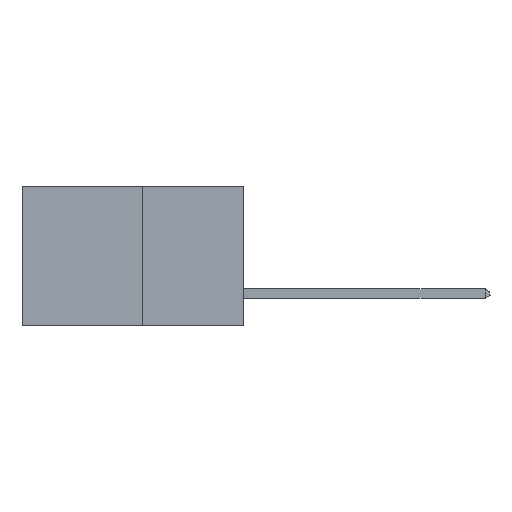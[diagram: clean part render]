
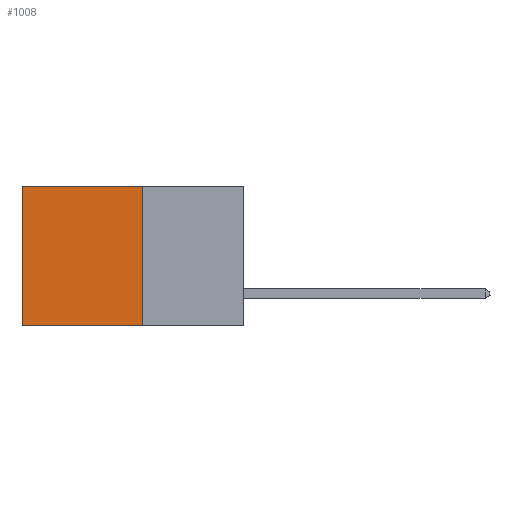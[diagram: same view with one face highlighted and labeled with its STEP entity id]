
A CAD part, left-side view. The second image highlights one B-rep face of the part: STEP entity #1008.
In plain terms, the highlighted planar face has unit normal (-1, 0, 0).
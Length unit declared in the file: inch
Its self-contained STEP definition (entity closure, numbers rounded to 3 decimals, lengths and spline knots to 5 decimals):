
#1008 = ADVANCED_FACE ( 'NONE', ( #6183 ), #26153, .F. ) ;
#1246 = DIRECTION ( 'NONE',  ( 0., 1., 0. ) ) ;
#1373 = CARTESIAN_POINT ( 'NONE',  ( 0.277, 0.59, -0.37 ) ) ;
#1601 = DIRECTION ( 'NONE',  ( 0., 0., -1. ) ) ;
#2388 = LINE ( 'NONE', #1373, #7312 ) ;
#3856 = CARTESIAN_POINT ( 'NONE',  ( 0.277, 0.27, -0.37 ) ) ;
#4188 = VECTOR ( 'NONE', #12572, 39.37008 ) ;
#4599 = EDGE_LOOP ( 'NONE', ( #15728, #17544, #7370, #18538 ) ) ;
#6183 = FACE_OUTER_BOUND ( 'NONE', #4599, .T. ) ;
#6371 = CARTESIAN_POINT ( 'NONE',  ( 0.277, 0.27, 0. ) ) ;
#6866 = EDGE_CURVE ( 'NONE', #22824, #24091, #2388, .T. ) ;
#7312 = VECTOR ( 'NONE', #1601, 39.37008 ) ;
#7370 = ORIENTED_EDGE ( 'NONE', *, *, #10725, .F. ) ;
#8289 = CARTESIAN_POINT ( 'NONE',  ( 0.277, 0.59, -0.37 ) ) ;
#8595 = LINE ( 'NONE', #25782, #23568 ) ;
#9756 = LINE ( 'NONE', #6371, #4188 ) ;
#10725 = EDGE_CURVE ( 'NONE', #12089, #18622, #21471, .T. ) ;
#12089 = VERTEX_POINT ( 'NONE', #15276 ) ;
#12447 = CARTESIAN_POINT ( 'NONE',  ( 0.277, 0.27, -0.37 ) ) ;
#12572 = DIRECTION ( 'NONE',  ( 0., 1., 0. ) ) ;
#15004 = EDGE_CURVE ( 'NONE', #18622, #24091, #8595, .T. ) ;
#15276 = CARTESIAN_POINT ( 'NONE',  ( 0.277, 0.27, 0. ) ) ;
#15728 = ORIENTED_EDGE ( 'NONE', *, *, #6866, .T. ) ;
#16427 = CARTESIAN_POINT ( 'NONE',  ( 0.277, 0.59, 0. ) ) ;
#17544 = ORIENTED_EDGE ( 'NONE', *, *, #15004, .F. ) ;
#18205 = DIRECTION ( 'NONE',  ( 0., 0., -1. ) ) ;
#18538 = ORIENTED_EDGE ( 'NONE', *, *, #26281, .T. ) ;
#18622 = VERTEX_POINT ( 'NONE', #19915 ) ;
#19915 = CARTESIAN_POINT ( 'NONE',  ( 0.277, 0.27, -0.37 ) ) ;
#21471 = LINE ( 'NONE', #3856, #22750 ) ;
#21568 = AXIS2_PLACEMENT_3D ( 'NONE', #12447, #26526, #18205 ) ;
#22750 = VECTOR ( 'NONE', #24391, 39.37008 ) ;
#22824 = VERTEX_POINT ( 'NONE', #16427 ) ;
#23568 = VECTOR ( 'NONE', #1246, 39.37008 ) ;
#24091 = VERTEX_POINT ( 'NONE', #8289 ) ;
#24391 = DIRECTION ( 'NONE',  ( 0., 0., -1. ) ) ;
#25782 = CARTESIAN_POINT ( 'NONE',  ( 0.277, 0.27, -0.37 ) ) ;
#26153 = PLANE ( 'NONE',  #21568 ) ;
#26281 = EDGE_CURVE ( 'NONE', #12089, #22824, #9756, .T. ) ;
#26526 = DIRECTION ( 'NONE',  ( 1., 0., 0. ) ) ;
